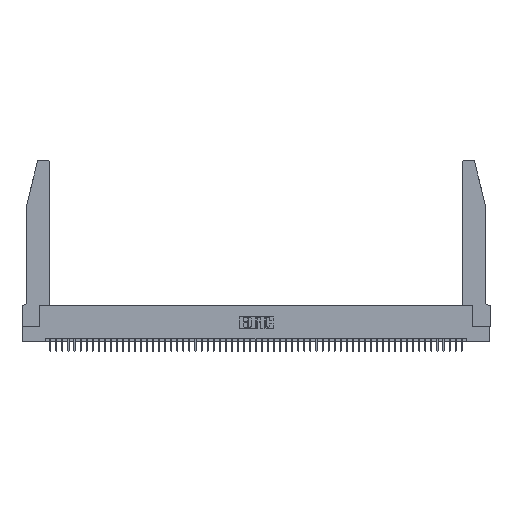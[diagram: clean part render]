
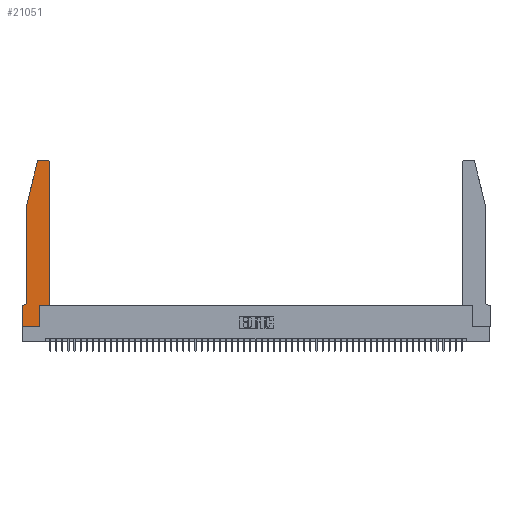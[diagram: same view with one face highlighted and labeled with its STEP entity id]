
A CAD part, top view. The second image highlights one B-rep face of the part: STEP entity #21051.
In plain terms, the highlighted planar face has unit normal (0, 0, 1).
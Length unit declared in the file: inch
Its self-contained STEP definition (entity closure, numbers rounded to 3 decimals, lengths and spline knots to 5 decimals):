
#183 = LINE ( 'NONE', #42613, #34964 ) ;
#219 = CARTESIAN_POINT ( 'NONE',  ( 0.4505, 0.35, 0.37 ) ) ;
#220 = CARTESIAN_POINT ( 'NONE',  ( 0.0055, 0.35, 0.37 ) ) ;
#482 = VECTOR ( 'NONE', #16552, 39.37008 ) ;
#2117 = EDGE_CURVE ( 'NONE', #43489, #3931, #6710, .T. ) ;
#3248 = VECTOR ( 'NONE', #44180, 39.37008 ) ;
#3507 = EDGE_CURVE ( 'NONE', #9089, #5185, #47317, .T. ) ;
#3931 = VERTEX_POINT ( 'NONE', #28669 ) ;
#4369 = DIRECTION ( 'NONE',  ( 0., 0., -1. ) ) ;
#5185 = VERTEX_POINT ( 'NONE', #35961 ) ;
#5949 = VERTEX_POINT ( 'NONE', #49156 ) ;
#6177 = EDGE_CURVE ( 'NONE', #39632, #11207, #183, .T. ) ;
#6634 = CARTESIAN_POINT ( 'NONE',  ( 0.0755, 2., 0.37 ) ) ;
#6710 = LINE ( 'NONE', #26355, #16157 ) ;
#6937 = LINE ( 'NONE', #22034, #10252 ) ;
#8900 = CARTESIAN_POINT ( 'NONE',  ( 0.0055, 0.42, 0.37 ) ) ;
#9089 = VERTEX_POINT ( 'NONE', #15704 ) ;
#9196 = AXIS2_PLACEMENT_3D ( 'NONE', #42453, #41900, #37945 ) ;
#9776 = ORIENTED_EDGE ( 'NONE', *, *, #45890, .T. ) ;
#10099 = CARTESIAN_POINT ( 'NONE',  ( 0.4205, 2.75, 0.37 ) ) ;
#10252 = VECTOR ( 'NONE', #52051, 39.37008 ) ;
#10713 = DIRECTION ( 'NONE',  ( 0., 1., 0. ) ) ;
#10847 = CARTESIAN_POINT ( 'NONE',  ( 0.284, 2.72, 0.37 ) ) ;
#10926 = AXIS2_PLACEMENT_3D ( 'NONE', #20478, #42120, #46756 ) ;
#10954 = VERTEX_POINT ( 'NONE', #220 ) ;
#11207 = VERTEX_POINT ( 'NONE', #40916 ) ;
#11835 = VECTOR ( 'NONE', #33952, 39.37008 ) ;
#11956 = PLANE ( 'NONE',  #9196 ) ;
#12561 = ORIENTED_EDGE ( 'NONE', *, *, #3507, .T. ) ;
#13240 = LINE ( 'NONE', #44562, #21304 ) ;
#15704 = CARTESIAN_POINT ( 'NONE',  ( 0.4505, 0.35, 0.37 ) ) ;
#15818 = CIRCLE ( 'NONE', #48346, 0.03 ) ;
#16157 = VECTOR ( 'NONE', #43125, 39.37008 ) ;
#16552 = DIRECTION ( 'NONE',  ( 0., 1., 0. ) ) ;
#16888 = EDGE_CURVE ( 'NONE', #11207, #10954, #48479, .T. ) ;
#18023 = EDGE_CURVE ( 'NONE', #5185, #43489, #29719, .T. ) ;
#18387 = EDGE_CURVE ( 'NONE', #46803, #9089, #19581, .T. ) ;
#19581 = LINE ( 'NONE', #35329, #52275 ) ;
#20085 = LINE ( 'NONE', #35946, #3248 ) ;
#20478 = CARTESIAN_POINT ( 'NONE',  ( 0.4205, 2.72, 0.37 ) ) ;
#20738 = FACE_OUTER_BOUND ( 'NONE', #34977, .T. ) ;
#21051 = ADVANCED_FACE ( 'NONE', ( #20738 ), #11956, .T. ) ;
#21304 = VECTOR ( 'NONE', #10713, 39.37008 ) ;
#21315 = VERTEX_POINT ( 'NONE', #44259 ) ;
#21917 = LINE ( 'NONE', #42915, #11835 ) ;
#22034 = CARTESIAN_POINT ( 'NONE',  ( 0., 0., 0.37 ) ) ;
#23251 = DIRECTION ( 'NONE',  ( 0., 0., 1. ) ) ;
#24441 = CARTESIAN_POINT ( 'NONE',  ( 0.25487, 2.72718, 0.37 ) ) ;
#24628 = VECTOR ( 'NONE', #33406, 39.37008 ) ;
#25959 = EDGE_CURVE ( 'NONE', #5949, #46803, #13240, .T. ) ;
#25961 = LINE ( 'NONE', #37511, #24628 ) ;
#26165 = VERTEX_POINT ( 'NONE', #24441 ) ;
#26355 = CARTESIAN_POINT ( 'NONE',  ( 0.2605, 2.75, 0.37 ) ) ;
#26620 = ORIENTED_EDGE ( 'NONE', *, *, #25959, .T. ) ;
#28575 = EDGE_CURVE ( 'NONE', #48514, #5949, #6937, .T. ) ;
#28669 = CARTESIAN_POINT ( 'NONE',  ( 0.284, 2.75, 0.37 ) ) ;
#28823 = CARTESIAN_POINT ( 'NONE',  ( 0.2865, 0.35, 0.37 ) ) ;
#29197 = ORIENTED_EDGE ( 'NONE', *, *, #38029, .T. ) ;
#29719 = CIRCLE ( 'NONE', #10926, 0.03 ) ;
#30762 = ORIENTED_EDGE ( 'NONE', *, *, #38021, .T. ) ;
#32711 = CARTESIAN_POINT ( 'NONE',  ( 0., 0., 0.37 ) ) ;
#32853 = ORIENTED_EDGE ( 'NONE', *, *, #47781, .T. ) ;
#33406 = DIRECTION ( 'NONE',  ( -1., 0., 0. ) ) ;
#33952 = DIRECTION ( 'NONE',  ( 0., -1., 0. ) ) ;
#34191 = ORIENTED_EDGE ( 'NONE', *, *, #16888, .T. ) ;
#34530 = DIRECTION ( 'NONE',  ( -1., 0., 0. ) ) ;
#34964 = VECTOR ( 'NONE', #38841, 39.37008 ) ;
#34977 = EDGE_LOOP ( 'NONE', ( #51336, #32853, #9776, #43804, #34191, #30762, #29197, #51130, #26620, #39461, #12561, #51746 ) ) ;
#35329 = CARTESIAN_POINT ( 'NONE',  ( 0.4505, 0.35, 0.37 ) ) ;
#35946 = CARTESIAN_POINT ( 'NONE',  ( 0.0755, 2., 0.37 ) ) ;
#35961 = CARTESIAN_POINT ( 'NONE',  ( 0.4505, 2.72, 0.37 ) ) ;
#37068 = AXIS2_PLACEMENT_3D ( 'NONE', #8900, #4369, #34530 ) ;
#37511 = CARTESIAN_POINT ( 'NONE',  ( 0.0755, 0.35, 0.37 ) ) ;
#37945 = DIRECTION ( 'NONE',  ( 1., 0., 0. ) ) ;
#38021 = EDGE_CURVE ( 'NONE', #10954, #21315, #25961, .T. ) ;
#38029 = EDGE_CURVE ( 'NONE', #21315, #48514, #21917, .T. ) ;
#38841 = DIRECTION ( 'NONE',  ( 0., -1., 0. ) ) ;
#39461 = ORIENTED_EDGE ( 'NONE', *, *, #18387, .T. ) ;
#39632 = VERTEX_POINT ( 'NONE', #6634 ) ;
#40916 = CARTESIAN_POINT ( 'NONE',  ( 0.0755, 0.42, 0.37 ) ) ;
#41900 = DIRECTION ( 'NONE',  ( 0., 0., 1. ) ) ;
#42120 = DIRECTION ( 'NONE',  ( 0., 0., 1. ) ) ;
#42453 = CARTESIAN_POINT ( 'NONE',  ( 0., 0.35, 0.37 ) ) ;
#42613 = CARTESIAN_POINT ( 'NONE',  ( 0.0755, 2., 0.37 ) ) ;
#42915 = CARTESIAN_POINT ( 'NONE',  ( 0., 0., 0.37 ) ) ;
#43125 = DIRECTION ( 'NONE',  ( -1., 0., 0. ) ) ;
#43489 = VERTEX_POINT ( 'NONE', #10099 ) ;
#43804 = ORIENTED_EDGE ( 'NONE', *, *, #6177, .T. ) ;
#44180 = DIRECTION ( 'NONE',  ( -0.239, -0.971, 0. ) ) ;
#44259 = CARTESIAN_POINT ( 'NONE',  ( 0., 0.35, 0.37 ) ) ;
#44562 = CARTESIAN_POINT ( 'NONE',  ( 0.2865, 0.35, 0.37 ) ) ;
#45236 = DIRECTION ( 'NONE',  ( 1., 0., 0. ) ) ;
#45890 = EDGE_CURVE ( 'NONE', #26165, #39632, #20085, .T. ) ;
#46756 = DIRECTION ( 'NONE',  ( 1., 0., 0. ) ) ;
#46803 = VERTEX_POINT ( 'NONE', #28823 ) ;
#47317 = LINE ( 'NONE', #219, #482 ) ;
#47781 = EDGE_CURVE ( 'NONE', #3931, #26165, #15818, .T. ) ;
#47852 = DIRECTION ( 'NONE',  ( 1., 0., 0. ) ) ;
#48346 = AXIS2_PLACEMENT_3D ( 'NONE', #10847, #23251, #45236 ) ;
#48479 = CIRCLE ( 'NONE', #37068, 0.07 ) ;
#48514 = VERTEX_POINT ( 'NONE', #32711 ) ;
#49156 = CARTESIAN_POINT ( 'NONE',  ( 0.2865, 0., 0.37 ) ) ;
#51130 = ORIENTED_EDGE ( 'NONE', *, *, #28575, .T. ) ;
#51336 = ORIENTED_EDGE ( 'NONE', *, *, #2117, .T. ) ;
#51746 = ORIENTED_EDGE ( 'NONE', *, *, #18023, .T. ) ;
#52051 = DIRECTION ( 'NONE',  ( 1., 0., 0. ) ) ;
#52275 = VECTOR ( 'NONE', #47852, 39.37008 ) ;
